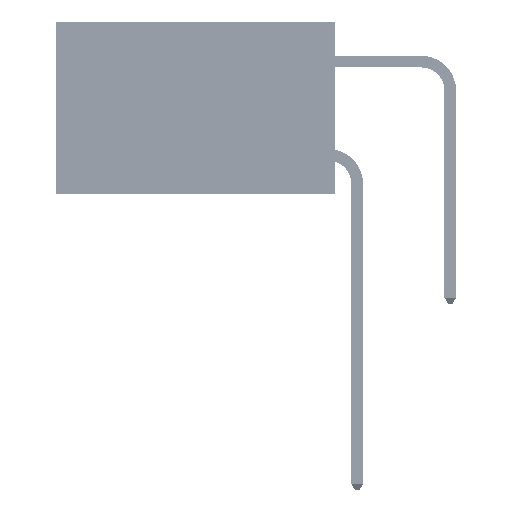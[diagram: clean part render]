
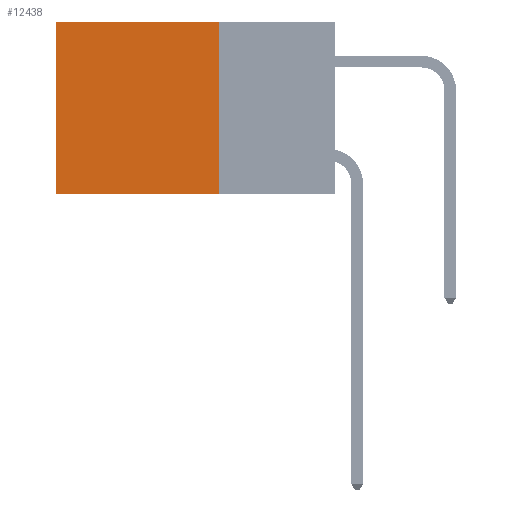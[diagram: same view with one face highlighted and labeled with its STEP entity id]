
A CAD part, left-side view. The second image highlights one B-rep face of the part: STEP entity #12438.
In plain terms, the highlighted planar face has unit normal (-1, 0, 0).
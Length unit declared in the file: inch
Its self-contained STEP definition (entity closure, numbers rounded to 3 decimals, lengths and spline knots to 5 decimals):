
#2744 = ORIENTED_EDGE ( 'NONE', *, *, #17673, .F. ) ;
#4583 = LINE ( 'NONE', #29687, #33429 ) ;
#6355 = CARTESIAN_POINT ( 'NONE',  ( 0.2875, 0.6, -0.37 ) ) ;
#9173 = EDGE_CURVE ( 'NONE', #49493, #21454, #41132, .T. ) ;
#10163 = ORIENTED_EDGE ( 'NONE', *, *, #9173, .T. ) ;
#10502 = PLANE ( 'NONE',  #15427 ) ;
#10553 = DIRECTION ( 'NONE',  ( 0., 1., 0. ) ) ;
#10602 = CARTESIAN_POINT ( 'NONE',  ( 0.2875, 0.25, 0. ) ) ;
#12438 = ADVANCED_FACE ( 'NONE', ( #35366 ), #10502, .F. ) ;
#15427 = AXIS2_PLACEMENT_3D ( 'NONE', #37983, #41893, #18442 ) ;
#16832 = VECTOR ( 'NONE', #30383, 39.37008 ) ;
#17395 = VERTEX_POINT ( 'NONE', #36732 ) ;
#17560 = EDGE_CURVE ( 'NONE', #41295, #21454, #4583, .T. ) ;
#17673 = EDGE_CURVE ( 'NONE', #17395, #41295, #27279, .T. ) ;
#18442 = DIRECTION ( 'NONE',  ( 0., 0., -1. ) ) ;
#19107 = LINE ( 'NONE', #45734, #38730 ) ;
#20105 = EDGE_CURVE ( 'NONE', #17395, #49493, #19107, .T. ) ;
#21454 = VERTEX_POINT ( 'NONE', #6355 ) ;
#26328 = EDGE_LOOP ( 'NONE', ( #10163, #27902, #2744, #41764 ) ) ;
#27196 = CARTESIAN_POINT ( 'NONE',  ( 0.2875, 0.6, 0. ) ) ;
#27279 = LINE ( 'NONE', #10602, #16832 ) ;
#27902 = ORIENTED_EDGE ( 'NONE', *, *, #17560, .F. ) ;
#29687 = CARTESIAN_POINT ( 'NONE',  ( 0.2875, 0.25, -0.37 ) ) ;
#30383 = DIRECTION ( 'NONE',  ( 0., 0., -1. ) ) ;
#31137 = DIRECTION ( 'NONE',  ( 0., 0., -1. ) ) ;
#33429 = VECTOR ( 'NONE', #33650, 39.37008 ) ;
#33605 = CARTESIAN_POINT ( 'NONE',  ( 0.2875, 0.6, 0. ) ) ;
#33650 = DIRECTION ( 'NONE',  ( 0., 1., 0. ) ) ;
#35366 = FACE_OUTER_BOUND ( 'NONE', #26328, .T. ) ;
#36732 = CARTESIAN_POINT ( 'NONE',  ( 0.2875, 0.25, 0. ) ) ;
#37983 = CARTESIAN_POINT ( 'NONE',  ( 0.2875, 0.25, 0. ) ) ;
#38730 = VECTOR ( 'NONE', #10553, 39.37008 ) ;
#41132 = LINE ( 'NONE', #27196, #49091 ) ;
#41295 = VERTEX_POINT ( 'NONE', #50619 ) ;
#41764 = ORIENTED_EDGE ( 'NONE', *, *, #20105, .T. ) ;
#41893 = DIRECTION ( 'NONE',  ( 1., 0., 0. ) ) ;
#45734 = CARTESIAN_POINT ( 'NONE',  ( 0.2875, 0.25, 0. ) ) ;
#49091 = VECTOR ( 'NONE', #31137, 39.37008 ) ;
#49493 = VERTEX_POINT ( 'NONE', #33605 ) ;
#50619 = CARTESIAN_POINT ( 'NONE',  ( 0.2875, 0.25, -0.37 ) ) ;
